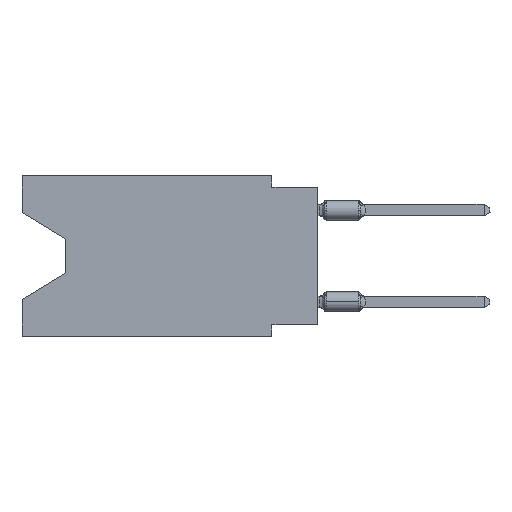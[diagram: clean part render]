
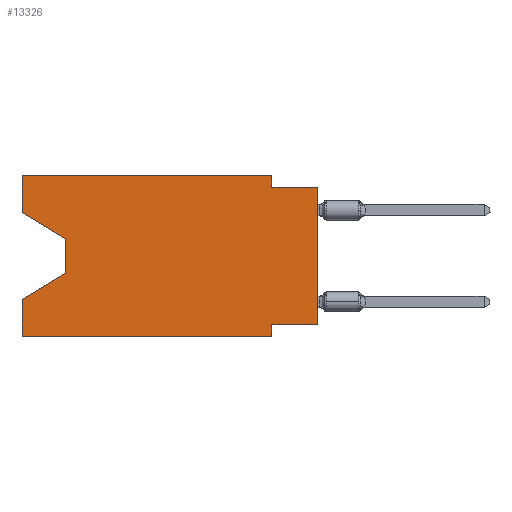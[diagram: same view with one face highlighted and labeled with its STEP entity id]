
A CAD part, left-side view. The second image highlights one B-rep face of the part: STEP entity #13326.
In plain terms, the highlighted planar face has unit normal (-1, 0, 0).
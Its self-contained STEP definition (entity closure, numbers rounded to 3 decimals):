
#265 = CARTESIAN_POINT ( 'NONE',  ( 0., 16.383, -2.038 ) ) ;
#642 = VERTEX_POINT ( 'NONE', #2384 ) ;
#891 = CARTESIAN_POINT ( 'NONE',  ( 0., 16.383, -8.89 ) ) ;
#1333 = VERTEX_POINT ( 'NONE', #29910 ) ;
#1654 = ORIENTED_EDGE ( 'NONE', *, *, #50308, .T. ) ;
#1924 = ORIENTED_EDGE ( 'NONE', *, *, #30483, .F. ) ;
#2209 = LINE ( 'NONE', #60836, #49214 ) ;
#2384 = CARTESIAN_POINT ( 'NONE',  ( 0., 16.383, -6.852 ) ) ;
#2757 = VERTEX_POINT ( 'NONE', #21691 ) ;
#2835 = CARTESIAN_POINT ( 'NONE',  ( 0., 0., -0.635 ) ) ;
#2933 = DIRECTION ( 'NONE',  ( 0., 0.855, -0.519 ) ) ;
#3138 = DIRECTION ( 'NONE',  ( 0., -1., 0. ) ) ;
#3817 = ORIENTED_EDGE ( 'NONE', *, *, #52631, .F. ) ;
#4310 = CARTESIAN_POINT ( 'NONE',  ( 0., 2.54, 0. ) ) ;
#4822 = ORIENTED_EDGE ( 'NONE', *, *, #15261, .F. ) ;
#5986 = DIRECTION ( 'NONE',  ( 0., 0., 1. ) ) ;
#6105 = DIRECTION ( 'NONE',  ( 1., 0., 0. ) ) ;
#7239 = CARTESIAN_POINT ( 'NONE',  ( 0., 2.54, -8.89 ) ) ;
#7398 = EDGE_CURVE ( 'NONE', #22022, #27717, #43060, .T. ) ;
#8035 = LINE ( 'NONE', #55843, #52297 ) ;
#8623 = VERTEX_POINT ( 'NONE', #12589 ) ;
#10452 = LINE ( 'NONE', #891, #20356 ) ;
#10461 = DIRECTION ( 'NONE',  ( 0., -0.855, -0.519 ) ) ;
#10778 = CARTESIAN_POINT ( 'NONE',  ( 0., 16.383, 0. ) ) ;
#11381 = DIRECTION ( 'NONE',  ( 0., 0., -1. ) ) ;
#11448 = DIRECTION ( 'NONE',  ( 0., -1., 0. ) ) ;
#12589 = CARTESIAN_POINT ( 'NONE',  ( 0., 13.97, -3.505 ) ) ;
#13326 = ADVANCED_FACE ( 'NONE', ( #39269 ), #34503, .F. ) ;
#14115 = CARTESIAN_POINT ( 'NONE',  ( 0., 0., -0.635 ) ) ;
#14329 = VERTEX_POINT ( 'NONE', #56830 ) ;
#15218 = EDGE_CURVE ( 'NONE', #44923, #1333, #2209, .T. ) ;
#15261 = EDGE_CURVE ( 'NONE', #33974, #27717, #60527, .T. ) ;
#15534 = LINE ( 'NONE', #10778, #18997 ) ;
#15731 = EDGE_CURVE ( 'NONE', #1333, #33974, #23477, .T. ) ;
#17668 = DIRECTION ( 'NONE',  ( 0., 1., 0. ) ) ;
#18574 = ORIENTED_EDGE ( 'NONE', *, *, #45020, .T. ) ;
#18997 = VECTOR ( 'NONE', #5986, 1000. ) ;
#20067 = VECTOR ( 'NONE', #58985, 1000. ) ;
#20152 = DIRECTION ( 'NONE',  ( 0., 0., -1. ) ) ;
#20356 = VECTOR ( 'NONE', #34684, 1000. ) ;
#21230 = CARTESIAN_POINT ( 'NONE',  ( 0., 0., -8.255 ) ) ;
#21691 = CARTESIAN_POINT ( 'NONE',  ( 0., 2.54, -8.255 ) ) ;
#21721 = VECTOR ( 'NONE', #11448, 1000. ) ;
#22022 = VERTEX_POINT ( 'NONE', #41537 ) ;
#23329 = ORIENTED_EDGE ( 'NONE', *, *, #7398, .T. ) ;
#23477 = LINE ( 'NONE', #4310, #32940 ) ;
#24547 = VECTOR ( 'NONE', #42870, 1000. ) ;
#25068 = CARTESIAN_POINT ( 'NONE',  ( 0., 16.383, -2.038 ) ) ;
#25930 = VECTOR ( 'NONE', #35935, 1000. ) ;
#26708 = LINE ( 'NONE', #46140, #25930 ) ;
#27685 = AXIS2_PLACEMENT_3D ( 'NONE', #53919, #6105, #20152 ) ;
#27717 = VERTEX_POINT ( 'NONE', #14115 ) ;
#29910 = CARTESIAN_POINT ( 'NONE',  ( 0., 2.54, 0. ) ) ;
#30123 = CARTESIAN_POINT ( 'NONE',  ( 0., 13.97, -5.385 ) ) ;
#30309 = VECTOR ( 'NONE', #17668, 1000. ) ;
#30483 = EDGE_CURVE ( 'NONE', #54398, #44923, #32073, .T. ) ;
#30550 = LINE ( 'NONE', #265, #44940 ) ;
#30808 = VERTEX_POINT ( 'NONE', #30123 ) ;
#32073 = LINE ( 'NONE', #32684, #24547 ) ;
#32364 = CARTESIAN_POINT ( 'NONE',  ( 0., 2.54, -0.635 ) ) ;
#32383 = ORIENTED_EDGE ( 'NONE', *, *, #42626, .F. ) ;
#32684 = CARTESIAN_POINT ( 'NONE',  ( 0., 16.383, 0. ) ) ;
#32940 = VECTOR ( 'NONE', #42575, 1000. ) ;
#33974 = VERTEX_POINT ( 'NONE', #32364 ) ;
#34503 = PLANE ( 'NONE',  #27685 ) ;
#34684 = DIRECTION ( 'NONE',  ( 0., -1., 0. ) ) ;
#34743 = EDGE_LOOP ( 'NONE', ( #18574, #1654, #44342, #3817, #58951, #32383, #38889, #23329, #4822, #49170, #49438, #1924 ) ) ;
#35478 = VERTEX_POINT ( 'NONE', #41241 ) ;
#35935 = DIRECTION ( 'NONE',  ( 0., 0., -1. ) ) ;
#38889 = ORIENTED_EDGE ( 'NONE', *, *, #59985, .F. ) ;
#39269 = FACE_OUTER_BOUND ( 'NONE', #34743, .T. ) ;
#39545 = CARTESIAN_POINT ( 'NONE',  ( 0., 0., 0. ) ) ;
#41241 = CARTESIAN_POINT ( 'NONE',  ( 0., 16.383, -8.89 ) ) ;
#41537 = CARTESIAN_POINT ( 'NONE',  ( 0., 0., -8.255 ) ) ;
#42575 = DIRECTION ( 'NONE',  ( 0., 0., -1. ) ) ;
#42626 = EDGE_CURVE ( 'NONE', #2757, #14329, #55038, .T. ) ;
#42870 = DIRECTION ( 'NONE',  ( 0., 0., 1. ) ) ;
#43060 = LINE ( 'NONE', #39545, #20067 ) ;
#44342 = ORIENTED_EDGE ( 'NONE', *, *, #49585, .T. ) ;
#44923 = VERTEX_POINT ( 'NONE', #59849 ) ;
#44940 = VECTOR ( 'NONE', #10461, 1000. ) ;
#45020 = EDGE_CURVE ( 'NONE', #54398, #8623, #30550, .T. ) ;
#45439 = LINE ( 'NONE', #21230, #30309 ) ;
#46140 = CARTESIAN_POINT ( 'NONE',  ( 0., 13.97, -3.505 ) ) ;
#49170 = ORIENTED_EDGE ( 'NONE', *, *, #15731, .F. ) ;
#49214 = VECTOR ( 'NONE', #3138, 1000. ) ;
#49438 = ORIENTED_EDGE ( 'NONE', *, *, #15218, .F. ) ;
#49585 = EDGE_CURVE ( 'NONE', #30808, #642, #8035, .T. ) ;
#50308 = EDGE_CURVE ( 'NONE', #8623, #30808, #26708, .T. ) ;
#52297 = VECTOR ( 'NONE', #2933, 1000. ) ;
#52631 = EDGE_CURVE ( 'NONE', #35478, #642, #15534, .T. ) ;
#53919 = CARTESIAN_POINT ( 'NONE',  ( 0., 16.383, 0. ) ) ;
#54398 = VERTEX_POINT ( 'NONE', #25068 ) ;
#55038 = LINE ( 'NONE', #7239, #59488 ) ;
#55843 = CARTESIAN_POINT ( 'NONE',  ( 0., 13.97, -5.385 ) ) ;
#56830 = CARTESIAN_POINT ( 'NONE',  ( 0., 2.54, -8.89 ) ) ;
#58010 = EDGE_CURVE ( 'NONE', #35478, #14329, #10452, .T. ) ;
#58951 = ORIENTED_EDGE ( 'NONE', *, *, #58010, .T. ) ;
#58985 = DIRECTION ( 'NONE',  ( 0., 0., 1. ) ) ;
#59488 = VECTOR ( 'NONE', #11381, 1000. ) ;
#59849 = CARTESIAN_POINT ( 'NONE',  ( 0., 16.383, 0. ) ) ;
#59985 = EDGE_CURVE ( 'NONE', #22022, #2757, #45439, .T. ) ;
#60527 = LINE ( 'NONE', #2835, #21721 ) ;
#60836 = CARTESIAN_POINT ( 'NONE',  ( 0., 16.383, 0. ) ) ;
